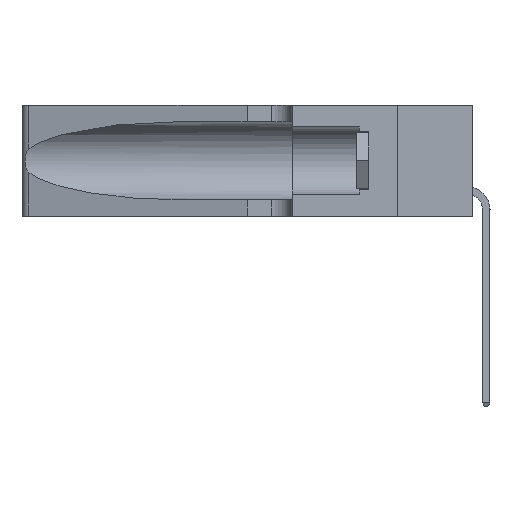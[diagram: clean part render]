
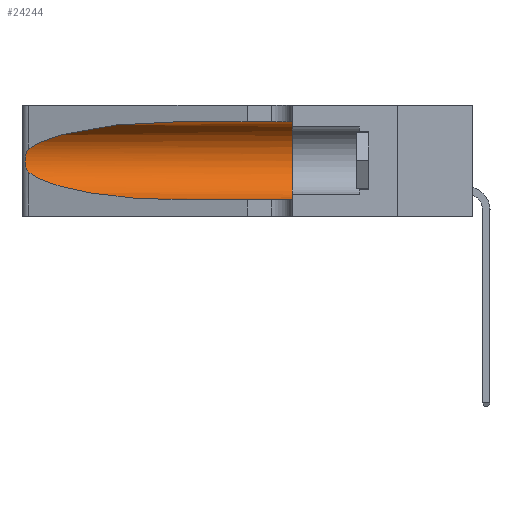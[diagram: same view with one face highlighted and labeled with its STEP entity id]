
A CAD part, left-side view. The second image highlights one B-rep face of the part: STEP entity #24244.
In plain terms, the highlighted cylindrical face has radius 3.308 mm (diameter 6.617 mm), a partial arc.
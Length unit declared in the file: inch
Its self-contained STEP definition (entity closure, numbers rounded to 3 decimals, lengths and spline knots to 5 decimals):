
#1144 = CARTESIAN_POINT ( 'NONE',  ( 0.25487, 1.22718, 0.14631 ) ) ;
#1420 = AXIS2_PLACEMENT_3D ( 'NONE', #35321, #27348, #11535 ) ;
#2544 = CARTESIAN_POINT ( 'NONE',  ( 0.1305, 0.35, 0.31525 ) ) ;
#3225 = DIRECTION ( 'NONE',  ( 0., 1., 0. ) ) ;
#3402 = DIRECTION ( 'NONE',  ( 0., 0., 1. ) ) ;
#5010 = CARTESIAN_POINT ( 'NONE',  ( 0.25856, 1.23593, 0.16098 ) ) ;
#6722 = CARTESIAN_POINT ( 'NONE',  ( 0.25487, 1.22718, 0.22369 ) ) ;
#6776 = VERTEX_POINT ( 'NONE', #28639 ) ;
#8502 =( BOUNDED_CURVE ( )  B_SPLINE_CURVE ( 3, ( #41609, #49690, #45556, #6722 ),
 .UNSPECIFIED., .F., .F. ) 
 B_SPLINE_CURVE_WITH_KNOTS ( ( 4, 4 ),
 ( 1.5708, 2.84003 ),
 .UNSPECIFIED. ) 
 CURVE ( )  GEOMETRIC_REPRESENTATION_ITEM ( )  RATIONAL_B_SPLINE_CURVE ( ( 1., 0.87, 0.87, 1. ) ) 
 REPRESENTATION_ITEM ( '' )  );
#8832 = CARTESIAN_POINT ( 'NONE',  ( 0.25854, 1.2359, 0.20912 ) ) ;
#8846 = CYLINDRICAL_SURFACE ( 'NONE', #1420, 0.13025 ) ;
#9878 = DIRECTION ( 'NONE',  ( 0., -1., 0. ) ) ;
#11535 = DIRECTION ( 'NONE',  ( 0., 0., -1. ) ) ;
#11870 = EDGE_CURVE ( 'NONE', #18999, #36529, #40386, .T. ) ;
#12801 = CARTESIAN_POINT ( 'NONE',  ( 0.26075, 1.23896, 0.19203 ) ) ;
#13300 = CARTESIAN_POINT ( 'NONE',  ( 0.25639, 1.23184, 0.21858 ) ) ;
#13468 = CARTESIAN_POINT ( 'NONE',  ( 0.25487, 1.22718, 0.22369 ) ) ;
#14068 = CARTESIAN_POINT ( 'NONE',  ( 0.18966, 0.96281, 0.05475 ) ) ;
#16747 = CARTESIAN_POINT ( 'NONE',  ( 0.26017, 1.23833, 0.17102 ) ) ;
#16917 = CARTESIAN_POINT ( 'NONE',  ( 0.25789, 1.23486, 0.15765 ) ) ;
#17505 = ORIENTED_EDGE ( 'NONE', *, *, #29578, .F. ) ;
#18170 = ORIENTED_EDGE ( 'NONE', *, *, #21134, .T. ) ;
#18999 = VERTEX_POINT ( 'NONE', #34886 ) ;
#20779 = LINE ( 'NONE', #29297, #28292 ) ;
#21134 = EDGE_CURVE ( 'NONE', #45922, #6776, #33910, .T. ) ;
#21792 =( BOUNDED_CURVE ( )  B_SPLINE_CURVE ( 3, ( #33656, #45340, #14068, #41963 ),
 .UNSPECIFIED., .F., .F. ) 
 B_SPLINE_CURVE_WITH_KNOTS ( ( 4, 4 ),
 ( 3.44316, 4.71239 ),
 .UNSPECIFIED. ) 
 CURVE ( )  GEOMETRIC_REPRESENTATION_ITEM ( )  RATIONAL_B_SPLINE_CURVE ( ( 1., 0.87, 0.87, 1. ) ) 
 REPRESENTATION_ITEM ( '' )  );
#22955 = CARTESIAN_POINT ( 'NONE',  ( 0.1305, 0.35, 0.185 ) ) ;
#24244 = ADVANCED_FACE ( 'NONE', ( #47866 ), #8846, .F. ) ;
#24956 = CARTESIAN_POINT ( 'NONE',  ( 0.25555, 1.22993, 0.14849 ) ) ;
#27348 = DIRECTION ( 'NONE',  ( 0., -1., 0. ) ) ;
#28292 = VECTOR ( 'NONE', #9878, 39.37008 ) ;
#28639 = CARTESIAN_POINT ( 'NONE',  ( 0.25487, 1.22718, 0.14631 ) ) ;
#29297 = CARTESIAN_POINT ( 'NONE',  ( 0.1305, 1.61858, 0.05475 ) ) ;
#29531 = CARTESIAN_POINT ( 'NONE',  ( 0.1305, 0.35, 0.05475 ) ) ;
#29578 = EDGE_CURVE ( 'NONE', #36529, #49248, #33479, .T. ) ;
#30923 = DIRECTION ( 'NONE',  ( 0., -1., 0. ) ) ;
#31095 = CARTESIAN_POINT ( 'NONE',  ( 0.1305, 1.61858, 0.31525 ) ) ;
#32584 = CARTESIAN_POINT ( 'NONE',  ( 0.25555, 1.22994, 0.2215 ) ) ;
#32817 = EDGE_CURVE ( 'NONE', #6776, #38992, #21792, .T. ) ;
#33321 = ORIENTED_EDGE ( 'NONE', *, *, #36486, .T. ) ;
#33479 = CIRCLE ( 'NONE', #41828, 0.13025 ) ;
#33656 = CARTESIAN_POINT ( 'NONE',  ( 0.25487, 1.22718, 0.14631 ) ) ;
#33910 = B_SPLINE_CURVE_WITH_KNOTS ( 'NONE', 3,
 ( #44268, #32584, #13300, #48548, #8832, #36561, #12801, #40538, #16747, #5010, #16917, #48383, #24956, #1144 ),
 .UNSPECIFIED., .F., .F.,
 ( 4, 2, 2, 2, 2, 2, 4 ),
 ( 0., 0.00027, 0.00053, 0.00107, 0.0016, 0.00187, 0.00214 ),
 .UNSPECIFIED. ) ;
#34886 = CARTESIAN_POINT ( 'NONE',  ( 0.1305, 0.72297, 0.31525 ) ) ;
#35321 = CARTESIAN_POINT ( 'NONE',  ( 0.1305, 1.61858, 0.185 ) ) ;
#36486 = EDGE_CURVE ( 'NONE', #18999, #45922, #8502, .T. ) ;
#36529 = VERTEX_POINT ( 'NONE', #2544 ) ;
#36561 = CARTESIAN_POINT ( 'NONE',  ( 0.26018, 1.23835, 0.19895 ) ) ;
#38896 = EDGE_CURVE ( 'NONE', #38992, #49248, #20779, .T. ) ;
#38992 = VERTEX_POINT ( 'NONE', #46250 ) ;
#39624 = ORIENTED_EDGE ( 'NONE', *, *, #11870, .F. ) ;
#39673 = ORIENTED_EDGE ( 'NONE', *, *, #32817, .T. ) ;
#40386 = LINE ( 'NONE', #31095, #42273 ) ;
#40497 = EDGE_LOOP ( 'NONE', ( #33321, #18170, #39673, #43884, #17505, #39624 ) ) ;
#40538 = CARTESIAN_POINT ( 'NONE',  ( 0.26075, 1.23896, 0.178 ) ) ;
#41609 = CARTESIAN_POINT ( 'NONE',  ( 0.1305, 0.72297, 0.31525 ) ) ;
#41828 = AXIS2_PLACEMENT_3D ( 'NONE', #22955, #3225, #3402 ) ;
#41963 = CARTESIAN_POINT ( 'NONE',  ( 0.1305, 0.72297, 0.05475 ) ) ;
#42273 = VECTOR ( 'NONE', #30923, 39.37008 ) ;
#43884 = ORIENTED_EDGE ( 'NONE', *, *, #38896, .T. ) ;
#44268 = CARTESIAN_POINT ( 'NONE',  ( 0.25487, 1.22718, 0.22369 ) ) ;
#45340 = CARTESIAN_POINT ( 'NONE',  ( 0.2373, 1.15595, 0.08982 ) ) ;
#45556 = CARTESIAN_POINT ( 'NONE',  ( 0.2373, 1.15595, 0.28018 ) ) ;
#45922 = VERTEX_POINT ( 'NONE', #13468 ) ;
#46250 = CARTESIAN_POINT ( 'NONE',  ( 0.1305, 0.72297, 0.05475 ) ) ;
#47866 = FACE_OUTER_BOUND ( 'NONE', #40497, .T. ) ;
#48383 = CARTESIAN_POINT ( 'NONE',  ( 0.25639, 1.23186, 0.15144 ) ) ;
#48548 = CARTESIAN_POINT ( 'NONE',  ( 0.25787, 1.23484, 0.2124 ) ) ;
#49248 = VERTEX_POINT ( 'NONE', #29531 ) ;
#49690 = CARTESIAN_POINT ( 'NONE',  ( 0.18966, 0.96281, 0.31525 ) ) ;
